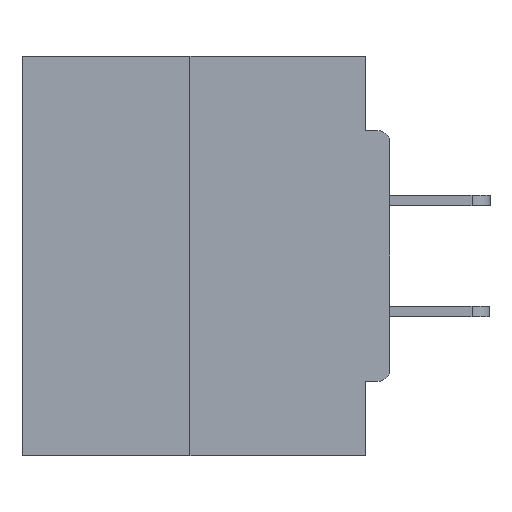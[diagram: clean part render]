
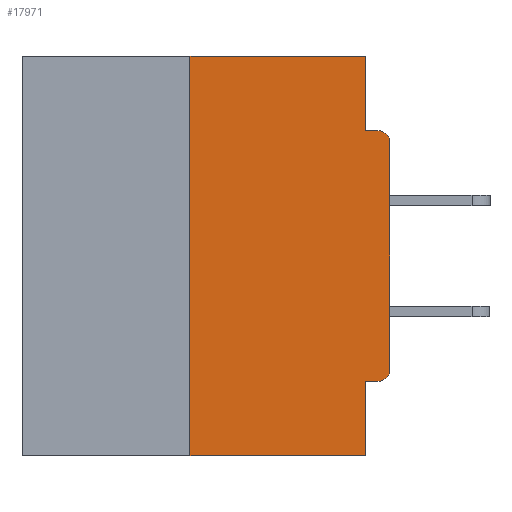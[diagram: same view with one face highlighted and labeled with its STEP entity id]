
A CAD part, left-side view. The second image highlights one B-rep face of the part: STEP entity #17971.
In plain terms, the highlighted planar face has unit normal (-1, 0, 0).
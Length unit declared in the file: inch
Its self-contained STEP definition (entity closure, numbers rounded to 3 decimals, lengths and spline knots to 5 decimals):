
#1033 = CARTESIAN_POINT ( 'NONE',  ( 0., 0.031, -0.4065 ) ) ;
#1487 = VERTEX_POINT ( 'NONE', #20986 ) ;
#1520 = ORIENTED_EDGE ( 'NONE', *, *, #3191, .T. ) ;
#2162 = LINE ( 'NONE', #6855, #4566 ) ;
#2359 = EDGE_CURVE ( 'NONE', #24279, #3516, #31013, .T. ) ;
#2430 = VECTOR ( 'NONE', #19247, 39.37008 ) ;
#2442 = DIRECTION ( 'NONE',  ( 0., -1., 0. ) ) ;
#2693 = ORIENTED_EDGE ( 'NONE', *, *, #21322, .T. ) ;
#3079 = CARTESIAN_POINT ( 'NONE',  ( 0., 0.015, -0.4065 ) ) ;
#3191 = EDGE_CURVE ( 'NONE', #6933, #26693, #4395, .T. ) ;
#3516 = VERTEX_POINT ( 'NONE', #4423 ) ;
#3893 = PLANE ( 'NONE',  #21962 ) ;
#4298 = CARTESIAN_POINT ( 'NONE',  ( 0., 0.031, 0. ) ) ;
#4395 = LINE ( 'NONE', #26921, #20061 ) ;
#4423 = CARTESIAN_POINT ( 'NONE',  ( 0., 0.031, -0.0935 ) ) ;
#4566 = VECTOR ( 'NONE', #30226, 39.37008 ) ;
#6128 = CARTESIAN_POINT ( 'NONE',  ( 0., 0.25, 0. ) ) ;
#6189 = DIRECTION ( 'NONE',  ( -1., 0., 0. ) ) ;
#6855 = CARTESIAN_POINT ( 'NONE',  ( 0., 0.46, 0. ) ) ;
#6933 = VERTEX_POINT ( 'NONE', #16274 ) ;
#7299 = CARTESIAN_POINT ( 'NONE',  ( 0., 0., -0.1085 ) ) ;
#8699 = LINE ( 'NONE', #24238, #31225 ) ;
#9407 = CIRCLE ( 'NONE', #23996, 0.015 ) ;
#9654 = FACE_OUTER_BOUND ( 'NONE', #14308, .T. ) ;
#9890 = DIRECTION ( 'NONE',  ( -1., 0., 0. ) ) ;
#10179 = VERTEX_POINT ( 'NONE', #3079 ) ;
#10269 = EDGE_CURVE ( 'NONE', #10179, #25335, #15738, .T. ) ;
#11548 = VECTOR ( 'NONE', #19073, 39.37008 ) ;
#11778 = VERTEX_POINT ( 'NONE', #6128 ) ;
#13150 = ORIENTED_EDGE ( 'NONE', *, *, #28478, .F. ) ;
#13248 = ORIENTED_EDGE ( 'NONE', *, *, #2359, .F. ) ;
#13328 = ORIENTED_EDGE ( 'NONE', *, *, #14821, .T. ) ;
#13792 = VECTOR ( 'NONE', #31549, 39.37008 ) ;
#14109 = DIRECTION ( 'NONE',  ( 0., 0., -1. ) ) ;
#14308 = EDGE_LOOP ( 'NONE', ( #25386, #20817, #1520, #13150, #31264, #29367, #13328, #2693, #30407, #13248 ) ) ;
#14342 = CARTESIAN_POINT ( 'NONE',  ( 0., 0.25, 0. ) ) ;
#14416 = CIRCLE ( 'NONE', #28432, 0.015 ) ;
#14638 = DIRECTION ( 'NONE',  ( 0., 0., -1. ) ) ;
#14821 = EDGE_CURVE ( 'NONE', #1487, #32264, #20598, .T. ) ;
#14860 = CARTESIAN_POINT ( 'NONE',  ( 0., 0.015, -0.0935 ) ) ;
#14950 = DIRECTION ( 'NONE',  ( 0., 0., -1. ) ) ;
#15738 = LINE ( 'NONE', #32183, #2430 ) ;
#15964 = VECTOR ( 'NONE', #2442, 39.37008 ) ;
#16274 = CARTESIAN_POINT ( 'NONE',  ( 0., 0.25, -0.5 ) ) ;
#17971 = ADVANCED_FACE ( 'NONE', ( #9654 ), #3893, .F. ) ;
#18334 = CARTESIAN_POINT ( 'NONE',  ( 0., 0.031, -0.5 ) ) ;
#19073 = DIRECTION ( 'NONE',  ( 0., 0., 1. ) ) ;
#19247 = DIRECTION ( 'NONE',  ( 0., 1., 0. ) ) ;
#20061 = VECTOR ( 'NONE', #32671, 39.37008 ) ;
#20598 = LINE ( 'NONE', #28935, #13792 ) ;
#20817 = ORIENTED_EDGE ( 'NONE', *, *, #28970, .F. ) ;
#20986 = CARTESIAN_POINT ( 'NONE',  ( 0., 0., -0.3915 ) ) ;
#21322 = EDGE_CURVE ( 'NONE', #32264, #26497, #9407, .T. ) ;
#21962 = AXIS2_PLACEMENT_3D ( 'NONE', #27027, #31888, #14109 ) ;
#22007 = DIRECTION ( 'NONE',  ( 0., 0., -1. ) ) ;
#23901 = EDGE_CURVE ( 'NONE', #11778, #24279, #2162, .T. ) ;
#23996 = AXIS2_PLACEMENT_3D ( 'NONE', #30011, #9890, #14950 ) ;
#24219 = CARTESIAN_POINT ( 'NONE',  ( 0., 0.031, 0. ) ) ;
#24238 = CARTESIAN_POINT ( 'NONE',  ( 0., 0.031, -0.5 ) ) ;
#24279 = VERTEX_POINT ( 'NONE', #24219 ) ;
#25335 = VERTEX_POINT ( 'NONE', #1033 ) ;
#25386 = ORIENTED_EDGE ( 'NONE', *, *, #23901, .F. ) ;
#25444 = CARTESIAN_POINT ( 'NONE',  ( 0., 0., -0.0935 ) ) ;
#26497 = VERTEX_POINT ( 'NONE', #14860 ) ;
#26635 = DIRECTION ( 'NONE',  ( 0., 0., -1. ) ) ;
#26693 = VERTEX_POINT ( 'NONE', #18334 ) ;
#26921 = CARTESIAN_POINT ( 'NONE',  ( 0., 0.46, -0.5 ) ) ;
#27027 = CARTESIAN_POINT ( 'NONE',  ( 0., 0.46, 0. ) ) ;
#27284 = EDGE_CURVE ( 'NONE', #10179, #1487, #14416, .T. ) ;
#27748 = VECTOR ( 'NONE', #14638, 39.37008 ) ;
#27934 = EDGE_CURVE ( 'NONE', #3516, #26497, #31270, .T. ) ;
#28432 = AXIS2_PLACEMENT_3D ( 'NONE', #29344, #6189, #22007 ) ;
#28478 = EDGE_CURVE ( 'NONE', #25335, #26693, #8699, .T. ) ;
#28935 = CARTESIAN_POINT ( 'NONE',  ( 0., 0., 0. ) ) ;
#28970 = EDGE_CURVE ( 'NONE', #6933, #11778, #32876, .T. ) ;
#29344 = CARTESIAN_POINT ( 'NONE',  ( 0., 0.015, -0.3915 ) ) ;
#29367 = ORIENTED_EDGE ( 'NONE', *, *, #27284, .T. ) ;
#30011 = CARTESIAN_POINT ( 'NONE',  ( 0., 0.015, -0.1085 ) ) ;
#30226 = DIRECTION ( 'NONE',  ( 0., -1., 0. ) ) ;
#30407 = ORIENTED_EDGE ( 'NONE', *, *, #27934, .F. ) ;
#31013 = LINE ( 'NONE', #4298, #27748 ) ;
#31225 = VECTOR ( 'NONE', #26635, 39.37008 ) ;
#31264 = ORIENTED_EDGE ( 'NONE', *, *, #10269, .F. ) ;
#31270 = LINE ( 'NONE', #25444, #15964 ) ;
#31549 = DIRECTION ( 'NONE',  ( 0., 0., 1. ) ) ;
#31888 = DIRECTION ( 'NONE',  ( 1., 0., 0. ) ) ;
#32183 = CARTESIAN_POINT ( 'NONE',  ( 0., 0., -0.4065 ) ) ;
#32264 = VERTEX_POINT ( 'NONE', #7299 ) ;
#32671 = DIRECTION ( 'NONE',  ( 0., -1., 0. ) ) ;
#32876 = LINE ( 'NONE', #14342, #11548 ) ;
